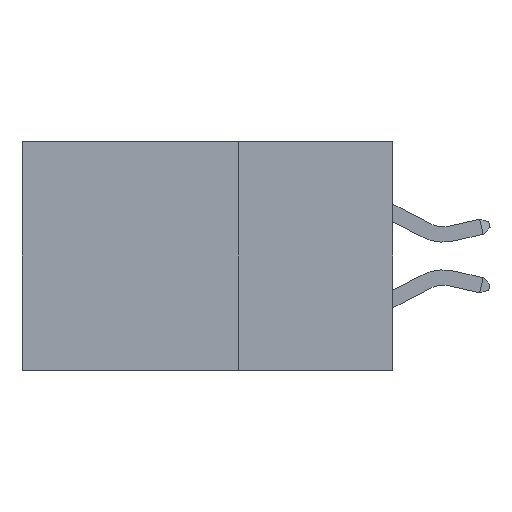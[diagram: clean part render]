
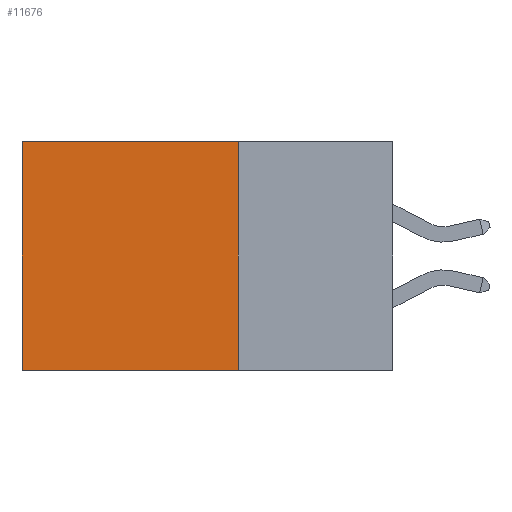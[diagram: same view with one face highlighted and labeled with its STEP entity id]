
A CAD part, left-side view. The second image highlights one B-rep face of the part: STEP entity #11676.
In plain terms, the highlighted planar face has unit normal (-1, 0, 0).
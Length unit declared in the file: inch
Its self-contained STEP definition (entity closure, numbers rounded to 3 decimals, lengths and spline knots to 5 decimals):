
#276 = DIRECTION ( 'NONE',  ( 0., 0., -1. ) ) ;
#282 = VERTEX_POINT ( 'NONE', #8419 ) ;
#320 = FACE_OUTER_BOUND ( 'NONE', #13022, .T. ) ;
#889 = EDGE_CURVE ( 'NONE', #6748, #7076, #6472, .T. ) ;
#2224 = VECTOR ( 'NONE', #6912, 39.37008 ) ;
#2937 = EDGE_CURVE ( 'NONE', #282, #6748, #9652, .T. ) ;
#3614 = DIRECTION ( 'NONE',  ( 0., 0., -1. ) ) ;
#5150 = EDGE_CURVE ( 'NONE', #12408, #7076, #6053, .T. ) ;
#5157 = ORIENTED_EDGE ( 'NONE', *, *, #5150, .T. ) ;
#5295 = CARTESIAN_POINT ( 'NONE',  ( 0.2875, 0.25, 0. ) ) ;
#5725 = CARTESIAN_POINT ( 'NONE',  ( 0.2875, 0.25, 0. ) ) ;
#5924 = CARTESIAN_POINT ( 'NONE',  ( 0.2875, 0.6, -0.37 ) ) ;
#6053 = LINE ( 'NONE', #14093, #11885 ) ;
#6150 = DIRECTION ( 'NONE',  ( 0., 1., 0. ) ) ;
#6445 = DIRECTION ( 'NONE',  ( 0., 0., -1. ) ) ;
#6472 = LINE ( 'NONE', #8744, #12631 ) ;
#6490 = CARTESIAN_POINT ( 'NONE',  ( 0.2875, 0.25, -0.37 ) ) ;
#6748 = VERTEX_POINT ( 'NONE', #6490 ) ;
#6912 = DIRECTION ( 'NONE',  ( 0., 1., 0. ) ) ;
#7076 = VERTEX_POINT ( 'NONE', #5924 ) ;
#8419 = CARTESIAN_POINT ( 'NONE',  ( 0.2875, 0.25, 0. ) ) ;
#8744 = CARTESIAN_POINT ( 'NONE',  ( 0.2875, 0.25, -0.37 ) ) ;
#8918 = VECTOR ( 'NONE', #3614, 39.37008 ) ;
#9282 = EDGE_CURVE ( 'NONE', #282, #12408, #14428, .T. ) ;
#9417 = AXIS2_PLACEMENT_3D ( 'NONE', #5295, #13339, #6445 ) ;
#9451 = CARTESIAN_POINT ( 'NONE',  ( 0.2875, 0.25, 0. ) ) ;
#9652 = LINE ( 'NONE', #9451, #8918 ) ;
#10123 = ORIENTED_EDGE ( 'NONE', *, *, #889, .F. ) ;
#11103 = PLANE ( 'NONE',  #9417 ) ;
#11237 = CARTESIAN_POINT ( 'NONE',  ( 0.2875, 0.6, 0. ) ) ;
#11676 = ADVANCED_FACE ( 'NONE', ( #320 ), #11103, .F. ) ;
#11885 = VECTOR ( 'NONE', #276, 39.37008 ) ;
#12408 = VERTEX_POINT ( 'NONE', #11237 ) ;
#12631 = VECTOR ( 'NONE', #6150, 39.37008 ) ;
#13022 = EDGE_LOOP ( 'NONE', ( #5157, #10123, #14513, #13947 ) ) ;
#13339 = DIRECTION ( 'NONE',  ( 1., 0., 0. ) ) ;
#13947 = ORIENTED_EDGE ( 'NONE', *, *, #9282, .T. ) ;
#14093 = CARTESIAN_POINT ( 'NONE',  ( 0.2875, 0.6, 0. ) ) ;
#14428 = LINE ( 'NONE', #5725, #2224 ) ;
#14513 = ORIENTED_EDGE ( 'NONE', *, *, #2937, .F. ) ;
